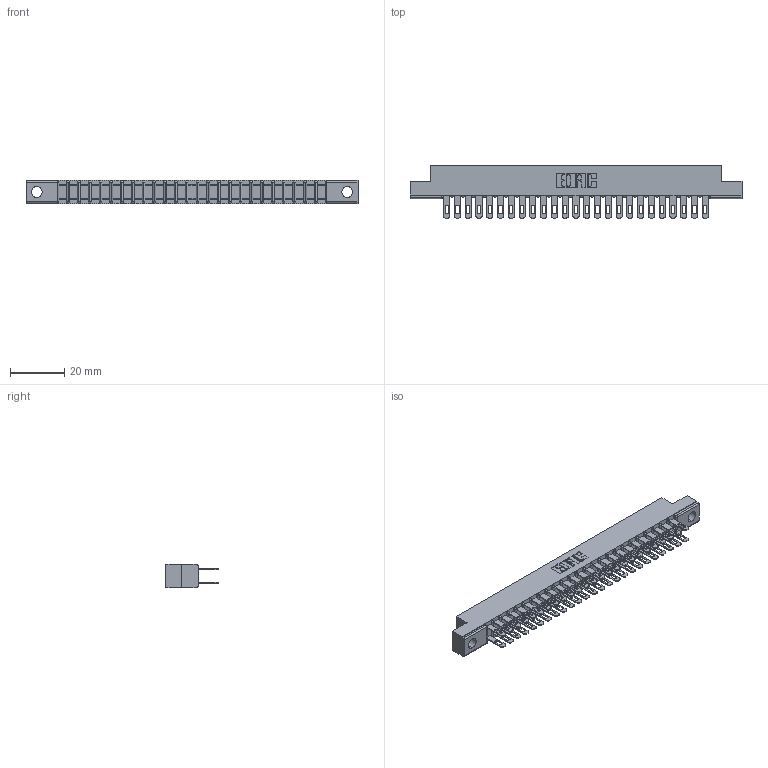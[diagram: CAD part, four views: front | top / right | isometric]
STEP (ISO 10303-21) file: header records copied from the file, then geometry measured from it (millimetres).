
FILE_DESCRIPTION (( 'STEP AP203' ), '1' );
FILE_NAME ('307-050-400-204.STEP', '2020-09-30T04:54:23', ( '' ), ( '' ), 'SwSTEP 2.0', 'SolidWorks 2020', '' );
FILE_SCHEMA (( 'CONFIG_CONTROL_DESIGN' ));
Length unit declared in the file: inch
Products named in the file (3): 307-050-400-204; 307 Part_.156 Dia Mounting Holes; 307-290-001_500
Assembly tree (51 placements, depth 2):
  307-050-400-204
    307 Part_.156 Dia Mounting Holes
    307-290-001_500  x50
Bounding box: 122.07 x 19.18 x 8.71 mm (x, y, z)
Volume: 8021.8 mm3; surface area: 15008.2 mm2
Topology: 51 solids, 51 shells, 2458 faces, 6859 edges, 4434 vertices
Faces by surface type: plane 1584, cylinder 822, sphere 52
Entity records: 24720 total; most frequent: CARTESIAN_POINT 4051, ORIENTED_EDGE 4010, DIRECTION 3969, EDGE_CURVE 2005, LINE 1537, VECTOR 1537, VERTEX_POINT 1298, AXIS2_PLACEMENT_3D 1216
